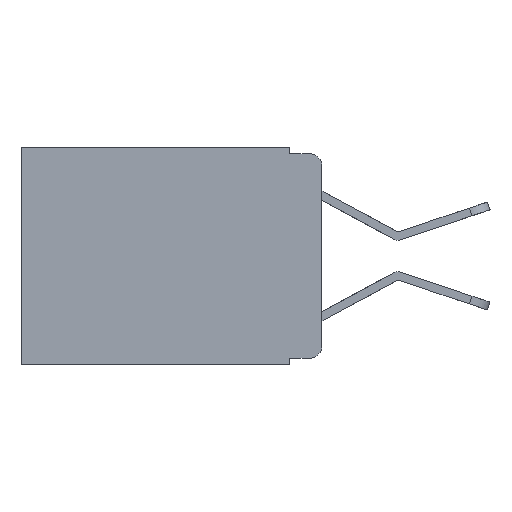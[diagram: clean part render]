
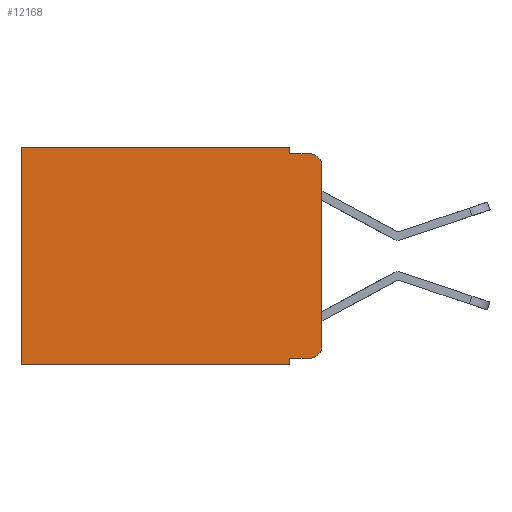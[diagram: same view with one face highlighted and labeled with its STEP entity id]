
A CAD part, left-side view. The second image highlights one B-rep face of the part: STEP entity #12168.
In plain terms, the highlighted planar face has unit normal (-1, 0, 0).
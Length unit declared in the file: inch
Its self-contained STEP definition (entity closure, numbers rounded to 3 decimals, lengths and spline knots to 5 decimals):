
#37 = CARTESIAN_POINT ( 'NONE',  ( 0.298, 0., -0.313 ) ) ;
#108 = EDGE_CURVE ( 'NONE', #2384, #5383, #8379, .T. ) ;
#590 = CARTESIAN_POINT ( 'NONE',  ( 0.298, 0.473, 0. ) ) ;
#642 = DIRECTION ( 'NONE',  ( 0., 0., -1. ) ) ;
#656 = LINE ( 'NONE', #2474, #6205 ) ;
#753 = ORIENTED_EDGE ( 'NONE', *, *, #6768, .F. ) ;
#1297 = VERTEX_POINT ( 'NONE', #8249 ) ;
#1617 = LINE ( 'NONE', #8372, #8651 ) ;
#2029 = AXIS2_PLACEMENT_3D ( 'NONE', #13200, #14393, #7289 ) ;
#2045 = DIRECTION ( 'NONE',  ( 0., 0., -1. ) ) ;
#2070 = LINE ( 'NONE', #590, #5123 ) ;
#2384 = VERTEX_POINT ( 'NONE', #13588 ) ;
#2474 = CARTESIAN_POINT ( 'NONE',  ( 0.298, 0.051, -0.333 ) ) ;
#2756 = EDGE_CURVE ( 'NONE', #8031, #6118, #1617, .T. ) ;
#2804 = ORIENTED_EDGE ( 'NONE', *, *, #2756, .F. ) ;
#3787 = CARTESIAN_POINT ( 'NONE',  ( 0.298, 0.051, 0. ) ) ;
#4471 = LINE ( 'NONE', #13700, #14017 ) ;
#4608 = VECTOR ( 'NONE', #4615, 39.37008 ) ;
#4615 = DIRECTION ( 'NONE',  ( 0., 1., 0. ) ) ;
#4686 = EDGE_CURVE ( 'NONE', #15194, #6118, #5399, .T. ) ;
#4699 = CARTESIAN_POINT ( 'NONE',  ( 0.298, 0.473, 0. ) ) ;
#4743 = EDGE_CURVE ( 'NONE', #7866, #1297, #10979, .T. ) ;
#4879 = PLANE ( 'NONE',  #2029 ) ;
#5105 = DIRECTION ( 'NONE',  ( 0., 0., -1. ) ) ;
#5123 = VECTOR ( 'NONE', #642, 39.37008 ) ;
#5383 = VERTEX_POINT ( 'NONE', #37 ) ;
#5399 = CIRCLE ( 'NONE', #12688, 0.02 ) ;
#5632 = CARTESIAN_POINT ( 'NONE',  ( 0.298, 0.02, -0.313 ) ) ;
#5777 = VERTEX_POINT ( 'NONE', #4699 ) ;
#6118 = VERTEX_POINT ( 'NONE', #8874 ) ;
#6205 = VECTOR ( 'NONE', #13411, 39.37008 ) ;
#6222 = VECTOR ( 'NONE', #13907, 39.37008 ) ;
#6565 = DIRECTION ( 'NONE',  ( 0., 1., 0. ) ) ;
#6768 = EDGE_CURVE ( 'NONE', #15194, #5383, #15519, .T. ) ;
#6781 = CARTESIAN_POINT ( 'NONE',  ( 0.298, 0.051, 0. ) ) ;
#6900 = CARTESIAN_POINT ( 'NONE',  ( 0.298, 0.02, -0.03 ) ) ;
#6920 = ORIENTED_EDGE ( 'NONE', *, *, #4743, .F. ) ;
#6965 = CARTESIAN_POINT ( 'NONE',  ( 0.298, 0.051, -0.333 ) ) ;
#7289 = DIRECTION ( 'NONE',  ( 0., 0., -1. ) ) ;
#7504 = EDGE_CURVE ( 'NONE', #10542, #7866, #13293, .T. ) ;
#7552 = EDGE_CURVE ( 'NONE', #5777, #1297, #2070, .T. ) ;
#7694 = ORIENTED_EDGE ( 'NONE', *, *, #13159, .T. ) ;
#7815 = EDGE_CURVE ( 'NONE', #10542, #2384, #656, .T. ) ;
#7866 = VERTEX_POINT ( 'NONE', #9933 ) ;
#7913 = ORIENTED_EDGE ( 'NONE', *, *, #108, .T. ) ;
#8031 = VERTEX_POINT ( 'NONE', #11440 ) ;
#8142 = DIRECTION ( 'NONE',  ( 0., 0., -1. ) ) ;
#8249 = CARTESIAN_POINT ( 'NONE',  ( 0.298, 0.473, -0.343 ) ) ;
#8266 = CARTESIAN_POINT ( 'NONE',  ( 0.298, 0.051, 0. ) ) ;
#8372 = CARTESIAN_POINT ( 'NONE',  ( 0.298, 0.051, -0.01 ) ) ;
#8379 = CIRCLE ( 'NONE', #12809, 0.02 ) ;
#8651 = VECTOR ( 'NONE', #15145, 39.37008 ) ;
#8874 = CARTESIAN_POINT ( 'NONE',  ( 0.298, 0.02, -0.01 ) ) ;
#9257 = VECTOR ( 'NONE', #13383, 39.37008 ) ;
#9853 = VERTEX_POINT ( 'NONE', #8266 ) ;
#9933 = CARTESIAN_POINT ( 'NONE',  ( 0.298, 0.051, -0.343 ) ) ;
#10082 = EDGE_CURVE ( 'NONE', #9853, #8031, #11270, .T. ) ;
#10218 = EDGE_LOOP ( 'NONE', ( #753, #13032, #2804, #15082, #7694, #13808, #6920, #13623, #13230, #7913 ) ) ;
#10542 = VERTEX_POINT ( 'NONE', #6965 ) ;
#10979 = LINE ( 'NONE', #15299, #4608 ) ;
#11270 = LINE ( 'NONE', #3787, #14070 ) ;
#11440 = CARTESIAN_POINT ( 'NONE',  ( 0.298, 0.051, -0.01 ) ) ;
#11967 = FACE_OUTER_BOUND ( 'NONE', #10218, .T. ) ;
#12168 = ADVANCED_FACE ( 'NONE', ( #11967 ), #4879, .F. ) ;
#12688 = AXIS2_PLACEMENT_3D ( 'NONE', #6900, #15201, #8142 ) ;
#12809 = AXIS2_PLACEMENT_3D ( 'NONE', #5632, #14597, #2045 ) ;
#13032 = ORIENTED_EDGE ( 'NONE', *, *, #4686, .T. ) ;
#13159 = EDGE_CURVE ( 'NONE', #9853, #5777, #4471, .T. ) ;
#13200 = CARTESIAN_POINT ( 'NONE',  ( 0.298, 0., 0. ) ) ;
#13230 = ORIENTED_EDGE ( 'NONE', *, *, #7815, .T. ) ;
#13293 = LINE ( 'NONE', #6781, #6222 ) ;
#13383 = DIRECTION ( 'NONE',  ( 0., 0., -1. ) ) ;
#13411 = DIRECTION ( 'NONE',  ( 0., -1., 0. ) ) ;
#13588 = CARTESIAN_POINT ( 'NONE',  ( 0.298, 0.02, -0.333 ) ) ;
#13623 = ORIENTED_EDGE ( 'NONE', *, *, #7504, .F. ) ;
#13700 = CARTESIAN_POINT ( 'NONE',  ( 0.298, 0., 0. ) ) ;
#13808 = ORIENTED_EDGE ( 'NONE', *, *, #7552, .T. ) ;
#13907 = DIRECTION ( 'NONE',  ( 0., 0., -1. ) ) ;
#14007 = CARTESIAN_POINT ( 'NONE',  ( 0.298, 0., -0.03 ) ) ;
#14017 = VECTOR ( 'NONE', #6565, 39.37008 ) ;
#14070 = VECTOR ( 'NONE', #5105, 39.37008 ) ;
#14393 = DIRECTION ( 'NONE',  ( 1., 0., 0. ) ) ;
#14578 = CARTESIAN_POINT ( 'NONE',  ( 0.298, 0., 0. ) ) ;
#14597 = DIRECTION ( 'NONE',  ( -1., 0., 0. ) ) ;
#15082 = ORIENTED_EDGE ( 'NONE', *, *, #10082, .F. ) ;
#15145 = DIRECTION ( 'NONE',  ( 0., -1., 0. ) ) ;
#15194 = VERTEX_POINT ( 'NONE', #14007 ) ;
#15201 = DIRECTION ( 'NONE',  ( -1., 0., 0. ) ) ;
#15299 = CARTESIAN_POINT ( 'NONE',  ( 0.298, 0., -0.343 ) ) ;
#15519 = LINE ( 'NONE', #14578, #9257 ) ;
